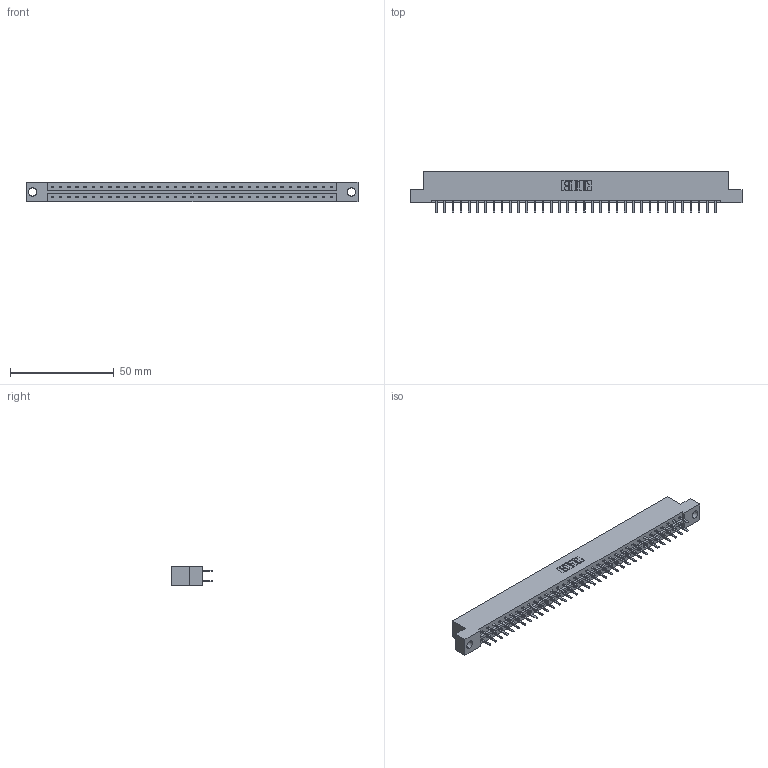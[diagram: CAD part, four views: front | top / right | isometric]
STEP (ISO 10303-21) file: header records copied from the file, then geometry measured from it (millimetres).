
FILE_DESCRIPTION (( 'STEP AP203' ), '1' );
FILE_NAME ('833-070-520-204.STEP', '2020-06-05T11:50:16', ( '' ), ( '' ), 'SwSTEP 2.0', 'SolidWorks 2020', '' );
FILE_SCHEMA (( 'CONFIG_CONTROL_DESIGN' ));
Length unit declared in the file: inch
Products named in the file (3): 345-292-001_345-293-120; 833-070-520-204; 833 Part_Flush - .156 Dia - TH
Assembly tree (71 placements, depth 2):
  833-070-520-204
    833 Part_Flush - .156 Dia - TH
    345-292-001_345-293-120  x70
Bounding box: 160.22 x 20.02 x 9.4 mm (x, y, z)
Volume: 16173.8 mm3; surface area: 18764.1 mm2
Topology: 71 solids, 71 shells, 4034 faces, 11721 edges, 7626 vertices
Faces by surface type: plane 2730, cylinder 1304
Entity records: 23539 total; most frequent: CARTESIAN_POINT 3922, ORIENTED_EDGE 3846, DIRECTION 3351, EDGE_CURVE 1923, LINE 1791, VECTOR 1791, VERTEX_POINT 1278, AXIS2_PLACEMENT_3D 780
